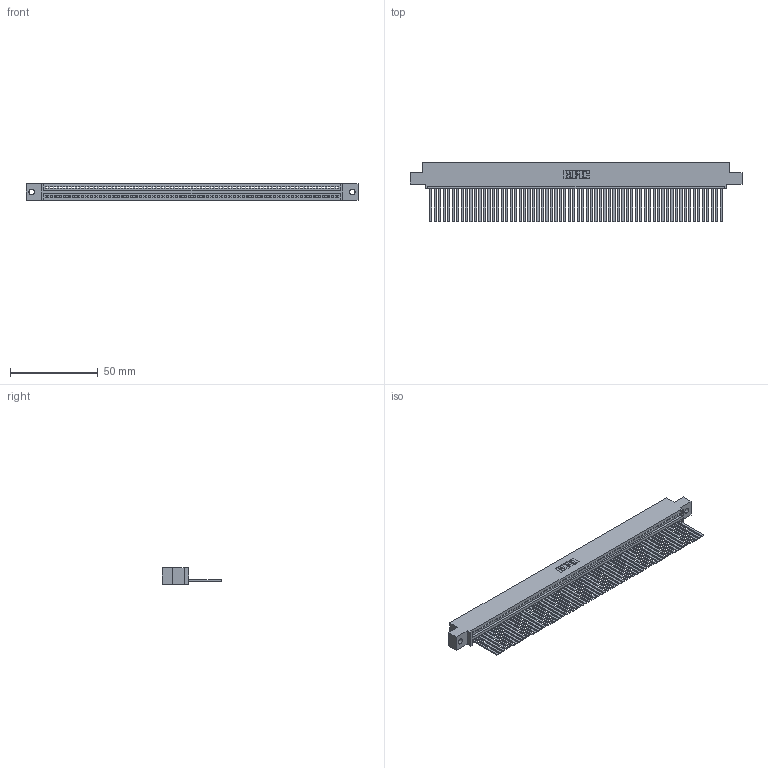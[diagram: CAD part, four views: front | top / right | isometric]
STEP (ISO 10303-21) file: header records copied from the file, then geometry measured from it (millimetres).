
FILE_DESCRIPTION (( 'STEP AP203' ), '1' );
FILE_NAME ('345-066-544-402.STEP', '2019-10-11T22:44:41', ( '' ), ( '' ), 'SwSTEP 2.0', 'SolidWorks 2016', '' );
FILE_SCHEMA (( 'CONFIG_CONTROL_DESIGN' ));
Length unit declared in the file: inch
Products named in the file (3): 345 Part_0.110 Offset - 0.128 Dia; 345-292-001_345-293-144; 345-066-544-402
Assembly tree (67 placements, depth 2):
  345-066-544-402
    345 Part_0.110 Offset - 0.128 Dia
    345-292-001_345-293-144  x66
Bounding box: 188.85 x 33.96 x 9.4 mm (x, y, z)
Volume: 18788 mm3; surface area: 27398.8 mm2
Topology: 67 solids, 67 shells, 3562 faces, 10781 edges, 7098 vertices
Faces by surface type: plane 2460, cylinder 1102
Entity records: 46393 total; most frequent: ORIENTED_EDGE 8042, CARTESIAN_POINT 8042, DIRECTION 6985, EDGE_CURVE 4021, LINE 3629, VECTOR 3629, VERTEX_POINT 2678, AXIS2_PLACEMENT_3D 1678
